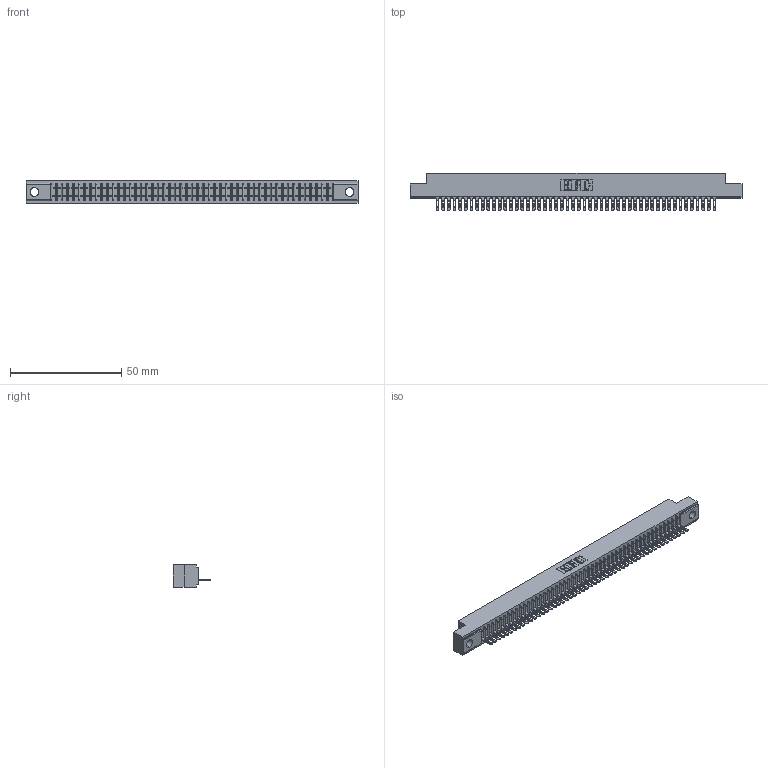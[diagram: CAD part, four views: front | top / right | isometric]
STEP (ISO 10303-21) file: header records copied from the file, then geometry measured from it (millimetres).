
FILE_DESCRIPTION (( 'STEP AP203' ), '1' );
FILE_NAME ('341-050-500-104.STEP', '2018-08-07T12:14:42', ( '' ), ( '' ), 'SwSTEP 2.0', 'SolidWorks 2016', '' );
FILE_SCHEMA (( 'CONFIG_CONTROL_DESIGN' ));
Length unit declared in the file: inch
Products named in the file (3): 341 Part_.156 (3.96) Dia Mounting Holes; 341-292-001_341-292-100; 341-050-500-104
Assembly tree (51 placements, depth 2):
  341-050-500-104
    341 Part_.156 (3.96) Dia Mounting Holes
    341-292-001_341-292-100  x50
Bounding box: 149.22 x 16.69 x 10.16 mm (x, y, z)
Volume: 10627.4 mm3; surface area: 16931 mm2
Topology: 51 solids, 51 shells, 4230 faces, 12202 edges, 7830 vertices
Faces by surface type: plane 2532, cylinder 1498, sphere 102, torus 98
Entity records: 58271 total; most frequent: CARTESIAN_POINT 9906, ORIENTED_EDGE 9892, DIRECTION 9552, EDGE_CURVE 4946, VECTOR 4008, LINE 4008, VERTEX_POINT 3126, AXIS2_PLACEMENT_3D 2772
